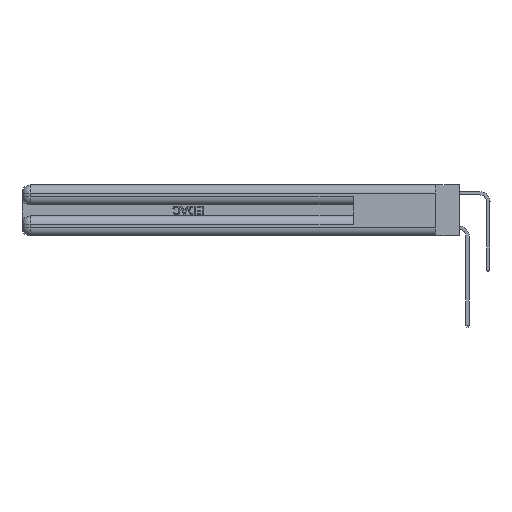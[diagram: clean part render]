
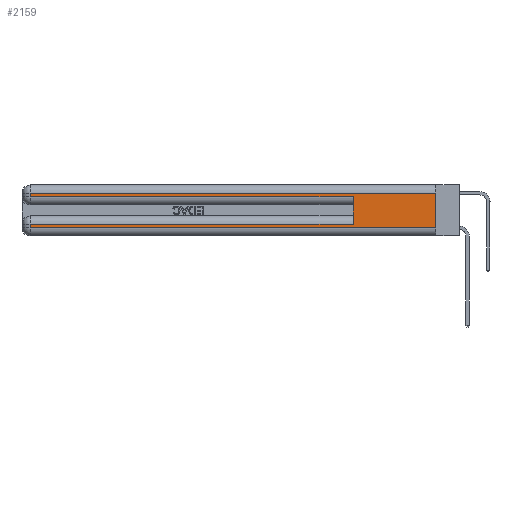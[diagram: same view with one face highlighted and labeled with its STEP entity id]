
A CAD part, left-side view. The second image highlights one B-rep face of the part: STEP entity #2159.
In plain terms, the highlighted planar face has unit normal (-1, 0, 0).
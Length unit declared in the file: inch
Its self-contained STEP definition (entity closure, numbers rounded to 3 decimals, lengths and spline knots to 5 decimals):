
#1093 = ORIENTED_EDGE ( 'NONE', *, *, #18972, .F. ) ;
#1737 = ORIENTED_EDGE ( 'NONE', *, *, #2893, .F. ) ;
#2159 = ADVANCED_FACE ( 'NONE', ( #5627 ), #20206, .F. ) ;
#2407 = EDGE_CURVE ( 'NONE', #8165, #27304, #8577, .T. ) ;
#2684 = LINE ( 'NONE', #17481, #22073 ) ;
#2893 = EDGE_CURVE ( 'NONE', #19050, #27304, #28702, .T. ) ;
#2980 = CARTESIAN_POINT ( 'NONE',  ( 0., 0., 0.285 ) ) ;
#3315 = EDGE_CURVE ( 'NONE', #8191, #16825, #2684, .T. ) ;
#4549 = CARTESIAN_POINT ( 'NONE',  ( 0., 0., 0.37 ) ) ;
#4998 = CARTESIAN_POINT ( 'NONE',  ( 0., 0.6, 0.085 ) ) ;
#5627 = FACE_OUTER_BOUND ( 'NONE', #20083, .T. ) ;
#6067 = VECTOR ( 'NONE', #32122, 39.37008 ) ;
#8165 = VERTEX_POINT ( 'NONE', #11725 ) ;
#8191 = VERTEX_POINT ( 'NONE', #17280 ) ;
#8577 = LINE ( 'NONE', #2980, #6067 ) ;
#9429 = ORIENTED_EDGE ( 'NONE', *, *, #18643, .T. ) ;
#10016 = CARTESIAN_POINT ( 'NONE',  ( 0., 0., 0.37 ) ) ;
#10235 = DIRECTION ( 'NONE',  ( 0., -1., 0. ) ) ;
#10817 = EDGE_CURVE ( 'NONE', #24986, #22757, #18916, .T. ) ;
#11069 = DIRECTION ( 'NONE',  ( 0., 0., -1. ) ) ;
#11350 = EDGE_CURVE ( 'NONE', #16520, #24986, #13532, .T. ) ;
#11725 = CARTESIAN_POINT ( 'NONE',  ( 0., 2.94, 0.285 ) ) ;
#13532 = LINE ( 'NONE', #18903, #30027 ) ;
#13811 = CARTESIAN_POINT ( 'NONE',  ( 0., 2.94, 0.37 ) ) ;
#13875 = EDGE_CURVE ( 'NONE', #19050, #16520, #31521, .T. ) ;
#14577 = CARTESIAN_POINT ( 'NONE',  ( 0., 2.94, 0.085 ) ) ;
#14689 = CARTESIAN_POINT ( 'NONE',  ( 0., 0., 0.06 ) ) ;
#14749 = VECTOR ( 'NONE', #26905, 39.37008 ) ;
#14762 = DIRECTION ( 'NONE',  ( 0., 0., -1. ) ) ;
#15506 = DIRECTION ( 'NONE',  ( 0., 0., -1. ) ) ;
#15722 = ORIENTED_EDGE ( 'NONE', *, *, #11350, .T. ) ;
#16520 = VERTEX_POINT ( 'NONE', #14577 ) ;
#16825 = VERTEX_POINT ( 'NONE', #21102 ) ;
#17280 = CARTESIAN_POINT ( 'NONE',  ( 0., 0., 0.31 ) ) ;
#17481 = CARTESIAN_POINT ( 'NONE',  ( 0., 0., 0.31 ) ) ;
#18643 = EDGE_CURVE ( 'NONE', #16825, #8165, #27170, .T. ) ;
#18855 = CARTESIAN_POINT ( 'NONE',  ( 0., 0.6, 0.145 ) ) ;
#18903 = CARTESIAN_POINT ( 'NONE',  ( 0., 2.94, 0.37 ) ) ;
#18916 = LINE ( 'NONE', #14689, #25498 ) ;
#18972 = EDGE_CURVE ( 'NONE', #8191, #22757, #30822, .T. ) ;
#19050 = VERTEX_POINT ( 'NONE', #4998 ) ;
#20083 = EDGE_LOOP ( 'NONE', ( #1093, #25184, #9429, #23604, #1737, #24161, #15722, #33694 ) ) ;
#20206 = PLANE ( 'NONE',  #25489 ) ;
#20569 = VECTOR ( 'NONE', #29477, 39.37008 ) ;
#21102 = CARTESIAN_POINT ( 'NONE',  ( 0., 2.94, 0.31 ) ) ;
#22073 = VECTOR ( 'NONE', #22735, 39.37008 ) ;
#22617 = VECTOR ( 'NONE', #14762, 39.37008 ) ;
#22735 = DIRECTION ( 'NONE',  ( 0., 1., 0. ) ) ;
#22757 = VERTEX_POINT ( 'NONE', #29215 ) ;
#23483 = CARTESIAN_POINT ( 'NONE',  ( 0., 2.94, 0.06 ) ) ;
#23604 = ORIENTED_EDGE ( 'NONE', *, *, #2407, .T. ) ;
#24161 = ORIENTED_EDGE ( 'NONE', *, *, #13875, .T. ) ;
#24986 = VERTEX_POINT ( 'NONE', #23483 ) ;
#25184 = ORIENTED_EDGE ( 'NONE', *, *, #3315, .T. ) ;
#25489 = AXIS2_PLACEMENT_3D ( 'NONE', #10016, #28568, #15506 ) ;
#25498 = VECTOR ( 'NONE', #10235, 39.37008 ) ;
#26905 = DIRECTION ( 'NONE',  ( 0., 0., 1. ) ) ;
#27060 = CARTESIAN_POINT ( 'NONE',  ( 0., 0., 0.085 ) ) ;
#27170 = LINE ( 'NONE', #13811, #20569 ) ;
#27304 = VERTEX_POINT ( 'NONE', #27686 ) ;
#27390 = DIRECTION ( 'NONE',  ( 0., 1., 0. ) ) ;
#27686 = CARTESIAN_POINT ( 'NONE',  ( 0., 0.6, 0.285 ) ) ;
#28250 = VECTOR ( 'NONE', #27390, 39.37008 ) ;
#28568 = DIRECTION ( 'NONE',  ( 1., 0., 0. ) ) ;
#28702 = LINE ( 'NONE', #18855, #14749 ) ;
#29215 = CARTESIAN_POINT ( 'NONE',  ( 0., 0., 0.06 ) ) ;
#29477 = DIRECTION ( 'NONE',  ( 0., 0., -1. ) ) ;
#30027 = VECTOR ( 'NONE', #11069, 39.37008 ) ;
#30822 = LINE ( 'NONE', #4549, #22617 ) ;
#31521 = LINE ( 'NONE', #27060, #28250 ) ;
#32122 = DIRECTION ( 'NONE',  ( 0., -1., 0. ) ) ;
#33694 = ORIENTED_EDGE ( 'NONE', *, *, #10817, .T. ) ;
